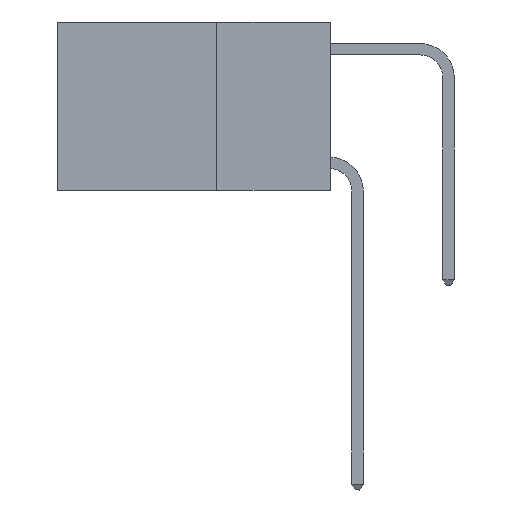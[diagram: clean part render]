
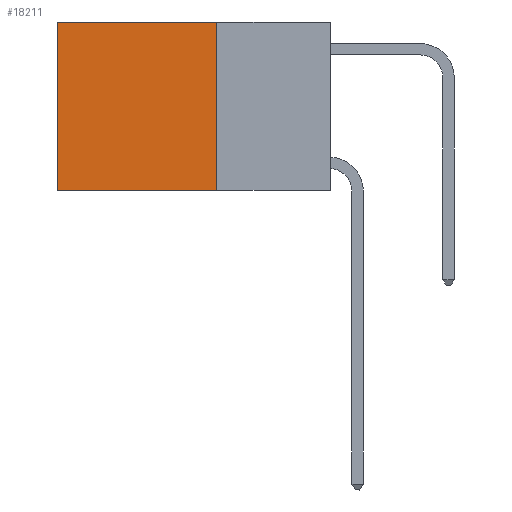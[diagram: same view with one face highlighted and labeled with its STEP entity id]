
A CAD part, left-side view. The second image highlights one B-rep face of the part: STEP entity #18211.
In plain terms, the highlighted planar face has unit normal (-1, 0, 0).
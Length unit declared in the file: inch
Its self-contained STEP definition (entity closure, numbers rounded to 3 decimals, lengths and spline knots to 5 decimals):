
#1479 = DIRECTION ( 'NONE',  ( 0., 0., -1. ) ) ;
#1864 = CARTESIAN_POINT ( 'NONE',  ( 0.2625, 0.25, 0. ) ) ;
#1965 = VECTOR ( 'NONE', #1479, 39.37008 ) ;
#2461 = ORIENTED_EDGE ( 'NONE', *, *, #7997, .F. ) ;
#3056 = CARTESIAN_POINT ( 'NONE',  ( 0.2625, 0.25, -0.37 ) ) ;
#3833 = DIRECTION ( 'NONE',  ( 1., 0., 0. ) ) ;
#3996 = VERTEX_POINT ( 'NONE', #1864 ) ;
#4835 = VERTEX_POINT ( 'NONE', #26333 ) ;
#6063 = AXIS2_PLACEMENT_3D ( 'NONE', #18100, #3833, #20529 ) ;
#6338 = CARTESIAN_POINT ( 'NONE',  ( 0.2625, 0.6, -0.37 ) ) ;
#7997 = EDGE_CURVE ( 'NONE', #3996, #19209, #21002, .T. ) ;
#9352 = LINE ( 'NONE', #26867, #23558 ) ;
#9841 = LINE ( 'NONE', #14031, #21816 ) ;
#10115 = ORIENTED_EDGE ( 'NONE', *, *, #16853, .T. ) ;
#11972 = EDGE_CURVE ( 'NONE', #19209, #18231, #9352, .T. ) ;
#12139 = VECTOR ( 'NONE', #29139, 39.37008 ) ;
#12422 = DIRECTION ( 'NONE',  ( 0., 1., 0. ) ) ;
#14031 = CARTESIAN_POINT ( 'NONE',  ( 0.2625, 0.6, 0. ) ) ;
#14332 = DIRECTION ( 'NONE',  ( 0., 0., -1. ) ) ;
#16853 = EDGE_CURVE ( 'NONE', #4835, #18231, #9841, .T. ) ;
#17657 = EDGE_CURVE ( 'NONE', #3996, #4835, #18506, .T. ) ;
#18100 = CARTESIAN_POINT ( 'NONE',  ( 0.2625, 0.25, 0. ) ) ;
#18211 = ADVANCED_FACE ( 'NONE', ( #18473 ), #30031, .F. ) ;
#18231 = VERTEX_POINT ( 'NONE', #6338 ) ;
#18473 = FACE_OUTER_BOUND ( 'NONE', #26652, .T. ) ;
#18506 = LINE ( 'NONE', #21936, #12139 ) ;
#19209 = VERTEX_POINT ( 'NONE', #3056 ) ;
#20529 = DIRECTION ( 'NONE',  ( 0., 0., -1. ) ) ;
#21002 = LINE ( 'NONE', #30062, #1965 ) ;
#21629 = ORIENTED_EDGE ( 'NONE', *, *, #11972, .F. ) ;
#21816 = VECTOR ( 'NONE', #14332, 39.37008 ) ;
#21936 = CARTESIAN_POINT ( 'NONE',  ( 0.2625, 0.25, 0. ) ) ;
#23558 = VECTOR ( 'NONE', #12422, 39.37008 ) ;
#26322 = ORIENTED_EDGE ( 'NONE', *, *, #17657, .T. ) ;
#26333 = CARTESIAN_POINT ( 'NONE',  ( 0.2625, 0.6, 0. ) ) ;
#26652 = EDGE_LOOP ( 'NONE', ( #10115, #21629, #2461, #26322 ) ) ;
#26867 = CARTESIAN_POINT ( 'NONE',  ( 0.2625, 0.25, -0.37 ) ) ;
#29139 = DIRECTION ( 'NONE',  ( 0., 1., 0. ) ) ;
#30031 = PLANE ( 'NONE',  #6063 ) ;
#30062 = CARTESIAN_POINT ( 'NONE',  ( 0.2625, 0.25, 0. ) ) ;
